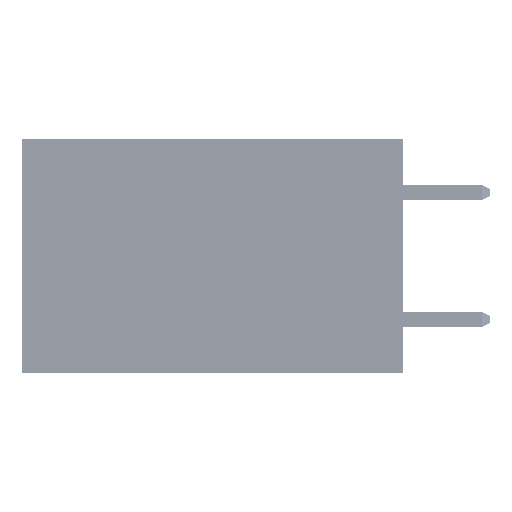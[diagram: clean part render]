
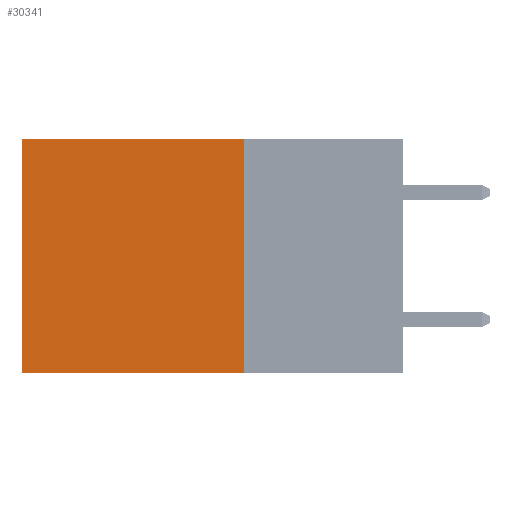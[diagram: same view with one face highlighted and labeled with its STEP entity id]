
A CAD part, left-side view. The second image highlights one B-rep face of the part: STEP entity #30341.
In plain terms, the highlighted planar face has unit normal (-1, 0, 0).
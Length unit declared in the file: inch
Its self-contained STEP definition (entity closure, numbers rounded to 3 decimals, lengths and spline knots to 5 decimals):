
#1689 = ORIENTED_EDGE ( 'NONE', *, *, #49713, .T. ) ;
#3271 = CARTESIAN_POINT ( 'NONE',  ( 0.2875, 0.25, -0.37 ) ) ;
#4604 = FACE_OUTER_BOUND ( 'NONE', #8998, .T. ) ;
#5969 = ORIENTED_EDGE ( 'NONE', *, *, #10507, .F. ) ;
#6355 = VERTEX_POINT ( 'NONE', #37269 ) ;
#8856 = VERTEX_POINT ( 'NONE', #3271 ) ;
#8998 = EDGE_LOOP ( 'NONE', ( #40918, #5969, #42077, #1689 ) ) ;
#9592 = DIRECTION ( 'NONE',  ( 0., 1., 0. ) ) ;
#10072 = VECTOR ( 'NONE', #22708, 39.37008 ) ;
#10173 = VECTOR ( 'NONE', #15189, 39.37008 ) ;
#10507 = EDGE_CURVE ( 'NONE', #8856, #11428, #45633, .T. ) ;
#11428 = VERTEX_POINT ( 'NONE', #24027 ) ;
#11956 = PLANE ( 'NONE',  #43624 ) ;
#12726 = CARTESIAN_POINT ( 'NONE',  ( 0.2875, 0.25, 0. ) ) ;
#14452 = EDGE_CURVE ( 'NONE', #6355, #8856, #26403, .T. ) ;
#15189 = DIRECTION ( 'NONE',  ( 0., 0., -1. ) ) ;
#18504 = VERTEX_POINT ( 'NONE', #27391 ) ;
#18568 = CARTESIAN_POINT ( 'NONE',  ( 0.2875, 0.25, 0. ) ) ;
#22708 = DIRECTION ( 'NONE',  ( 0., 0., -1. ) ) ;
#24027 = CARTESIAN_POINT ( 'NONE',  ( 0.2875, 0.6, -0.37 ) ) ;
#24290 = VECTOR ( 'NONE', #42594, 39.37008 ) ;
#25504 = CARTESIAN_POINT ( 'NONE',  ( 0.2875, 0.25, -0.37 ) ) ;
#26403 = LINE ( 'NONE', #42356, #10173 ) ;
#27391 = CARTESIAN_POINT ( 'NONE',  ( 0.2875, 0.6, 0. ) ) ;
#29499 = LINE ( 'NONE', #45453, #10072 ) ;
#30024 = VECTOR ( 'NONE', #9592, 39.37008 ) ;
#30341 = ADVANCED_FACE ( 'NONE', ( #4604 ), #11956, .F. ) ;
#31509 = DIRECTION ( 'NONE',  ( 0., 0., -1. ) ) ;
#37269 = CARTESIAN_POINT ( 'NONE',  ( 0.2875, 0.25, 0. ) ) ;
#38391 = LINE ( 'NONE', #18568, #24290 ) ;
#40918 = ORIENTED_EDGE ( 'NONE', *, *, #47196, .T. ) ;
#42077 = ORIENTED_EDGE ( 'NONE', *, *, #14452, .F. ) ;
#42356 = CARTESIAN_POINT ( 'NONE',  ( 0.2875, 0.25, 0. ) ) ;
#42594 = DIRECTION ( 'NONE',  ( 0., 1., 0. ) ) ;
#43624 = AXIS2_PLACEMENT_3D ( 'NONE', #12726, #44328, #31509 ) ;
#44328 = DIRECTION ( 'NONE',  ( 1., 0., 0. ) ) ;
#45453 = CARTESIAN_POINT ( 'NONE',  ( 0.2875, 0.6, 0. ) ) ;
#45633 = LINE ( 'NONE', #25504, #30024 ) ;
#47196 = EDGE_CURVE ( 'NONE', #18504, #11428, #29499, .T. ) ;
#49713 = EDGE_CURVE ( 'NONE', #6355, #18504, #38391, .T. ) ;
